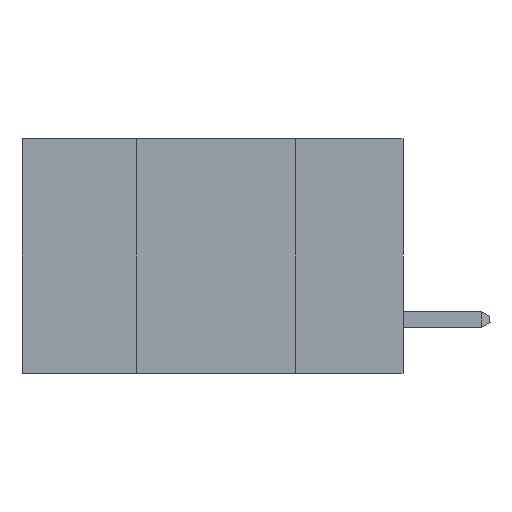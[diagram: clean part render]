
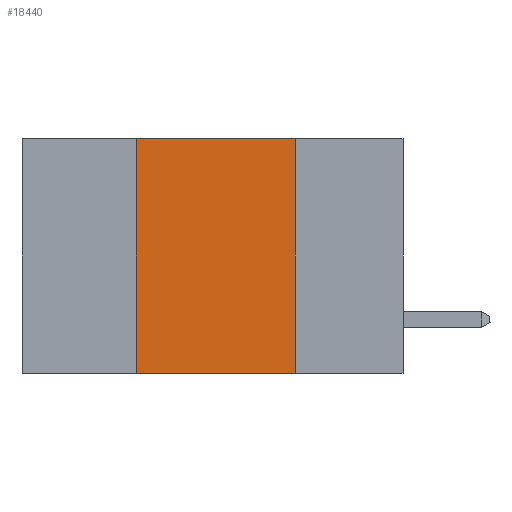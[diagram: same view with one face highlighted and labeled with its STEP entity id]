
A CAD part, left-side view. The second image highlights one B-rep face of the part: STEP entity #18440.
In plain terms, the highlighted planar face has unit normal (-1, 0, 0).
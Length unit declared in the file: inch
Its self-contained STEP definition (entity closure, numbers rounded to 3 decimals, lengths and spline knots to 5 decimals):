
#516 = VECTOR ( 'NONE', #19066, 39.37008 ) ;
#1175 = CARTESIAN_POINT ( 'NONE',  ( 0., 0.6, -0.37 ) ) ;
#2180 = VERTEX_POINT ( 'NONE', #15783 ) ;
#3213 = LINE ( 'NONE', #24573, #516 ) ;
#3767 = DIRECTION ( 'NONE',  ( 0., 0., 1. ) ) ;
#4125 = LINE ( 'NONE', #20877, #32032 ) ;
#4689 = CARTESIAN_POINT ( 'NONE',  ( 0., 0.17, 0. ) ) ;
#5610 = CARTESIAN_POINT ( 'NONE',  ( 0., 0.17, -0.37 ) ) ;
#7467 = LINE ( 'NONE', #34574, #32290 ) ;
#9028 = CARTESIAN_POINT ( 'NONE',  ( 0., 0.6, 0. ) ) ;
#9802 = ORIENTED_EDGE ( 'NONE', *, *, #27957, .F. ) ;
#10324 = EDGE_CURVE ( 'NONE', #13416, #34822, #3213, .T. ) ;
#10648 = EDGE_CURVE ( 'NONE', #11032, #34822, #15492, .T. ) ;
#11032 = VERTEX_POINT ( 'NONE', #34001 ) ;
#11288 = ORIENTED_EDGE ( 'NONE', *, *, #10324, .F. ) ;
#13416 = VERTEX_POINT ( 'NONE', #4689 ) ;
#15492 = LINE ( 'NONE', #1175, #24917 ) ;
#15783 = CARTESIAN_POINT ( 'NONE',  ( 0., 0.42, 0. ) ) ;
#18115 = DIRECTION ( 'NONE',  ( 0., -1., 0. ) ) ;
#18440 = ADVANCED_FACE ( 'NONE', ( #21994 ), #20430, .F. ) ;
#19066 = DIRECTION ( 'NONE',  ( 0., 0., -1. ) ) ;
#20430 = PLANE ( 'NONE',  #33609 ) ;
#20877 = CARTESIAN_POINT ( 'NONE',  ( 0., 0.6, 0. ) ) ;
#21994 = FACE_OUTER_BOUND ( 'NONE', #27093, .T. ) ;
#23808 = ORIENTED_EDGE ( 'NONE', *, *, #10648, .T. ) ;
#24573 = CARTESIAN_POINT ( 'NONE',  ( 0., 0.17, 0. ) ) ;
#24917 = VECTOR ( 'NONE', #18115, 39.37008 ) ;
#26260 = DIRECTION ( 'NONE',  ( 0., 0., -1. ) ) ;
#27093 = EDGE_LOOP ( 'NONE', ( #11288, #32308, #9802, #23808 ) ) ;
#27957 = EDGE_CURVE ( 'NONE', #11032, #2180, #7467, .T. ) ;
#28881 = DIRECTION ( 'NONE',  ( 1., 0., 0. ) ) ;
#32032 = VECTOR ( 'NONE', #35132, 39.37008 ) ;
#32290 = VECTOR ( 'NONE', #3767, 39.37008 ) ;
#32308 = ORIENTED_EDGE ( 'NONE', *, *, #35685, .F. ) ;
#33609 = AXIS2_PLACEMENT_3D ( 'NONE', #9028, #28881, #26260 ) ;
#34001 = CARTESIAN_POINT ( 'NONE',  ( 0., 0.42, -0.37 ) ) ;
#34574 = CARTESIAN_POINT ( 'NONE',  ( 0., 0.42, 0. ) ) ;
#34822 = VERTEX_POINT ( 'NONE', #5610 ) ;
#35132 = DIRECTION ( 'NONE',  ( 0., -1., 0. ) ) ;
#35685 = EDGE_CURVE ( 'NONE', #2180, #13416, #4125, .T. ) ;
